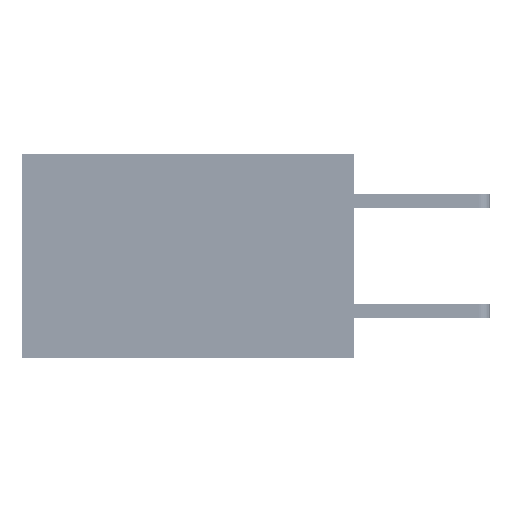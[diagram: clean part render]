
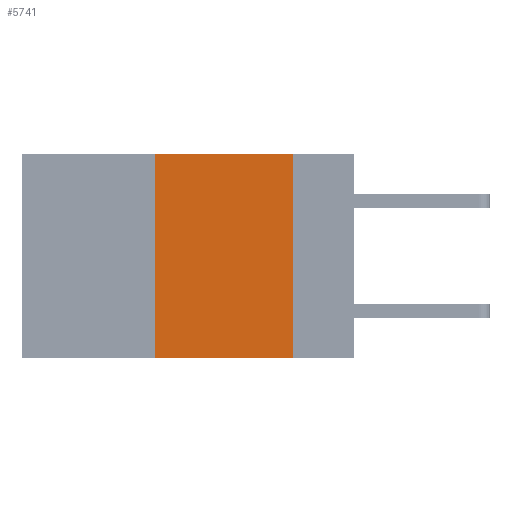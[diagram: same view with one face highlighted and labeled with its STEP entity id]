
A CAD part, left-side view. The second image highlights one B-rep face of the part: STEP entity #5741.
In plain terms, the highlighted planar face has unit normal (-1, 0, 0).
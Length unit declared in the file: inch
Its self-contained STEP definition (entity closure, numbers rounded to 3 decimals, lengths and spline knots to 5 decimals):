
#318 = EDGE_CURVE ( 'NONE', #2226, #13308, #30895, .T. ) ;
#563 = FACE_OUTER_BOUND ( 'NONE', #6860, .T. ) ;
#1146 = CARTESIAN_POINT ( 'NONE',  ( 0., 0.11, 0. ) ) ;
#2070 = AXIS2_PLACEMENT_3D ( 'NONE', #8874, #25288, #28802 ) ;
#2226 = VERTEX_POINT ( 'NONE', #36216 ) ;
#4583 = LINE ( 'NONE', #12927, #40667 ) ;
#5711 = ORIENTED_EDGE ( 'NONE', *, *, #24174, .T. ) ;
#5741 = ADVANCED_FACE ( 'NONE', ( #563 ), #32286, .F. ) ;
#6860 = EDGE_LOOP ( 'NONE', ( #35688, #47571, #44228, #5711 ) ) ;
#8874 = CARTESIAN_POINT ( 'NONE',  ( 0., 0.6, 0. ) ) ;
#10794 = CARTESIAN_POINT ( 'NONE',  ( 0., 0.11, -0.37 ) ) ;
#12927 = CARTESIAN_POINT ( 'NONE',  ( 0., 0.6, -0.37 ) ) ;
#13308 = VERTEX_POINT ( 'NONE', #1146 ) ;
#15041 = DIRECTION ( 'NONE',  ( 0., 0., 1. ) ) ;
#18506 = CARTESIAN_POINT ( 'NONE',  ( 0., 0.36, -0.37 ) ) ;
#19337 = CARTESIAN_POINT ( 'NONE',  ( 0., 0.6, 0. ) ) ;
#20428 = VECTOR ( 'NONE', #29364, 39.37008 ) ;
#24174 = EDGE_CURVE ( 'NONE', #38677, #51711, #4583, .T. ) ;
#24541 = EDGE_CURVE ( 'NONE', #38677, #2226, #27924, .T. ) ;
#25288 = DIRECTION ( 'NONE',  ( 1., 0., 0. ) ) ;
#27020 = EDGE_CURVE ( 'NONE', #13308, #51711, #49791, .T. ) ;
#27924 = LINE ( 'NONE', #35458, #31139 ) ;
#28802 = DIRECTION ( 'NONE',  ( 0., 0., -1. ) ) ;
#29364 = DIRECTION ( 'NONE',  ( 0., 0., -1. ) ) ;
#29579 = DIRECTION ( 'NONE',  ( 0., -1., 0. ) ) ;
#30895 = LINE ( 'NONE', #19337, #51021 ) ;
#31139 = VECTOR ( 'NONE', #15041, 39.37008 ) ;
#32286 = PLANE ( 'NONE',  #2070 ) ;
#35458 = CARTESIAN_POINT ( 'NONE',  ( 0., 0.36, 0. ) ) ;
#35688 = ORIENTED_EDGE ( 'NONE', *, *, #27020, .F. ) ;
#36216 = CARTESIAN_POINT ( 'NONE',  ( 0., 0.36, 0. ) ) ;
#38677 = VERTEX_POINT ( 'NONE', #18506 ) ;
#40667 = VECTOR ( 'NONE', #29579, 39.37008 ) ;
#41990 = CARTESIAN_POINT ( 'NONE',  ( 0., 0.11, 0. ) ) ;
#44228 = ORIENTED_EDGE ( 'NONE', *, *, #24541, .F. ) ;
#47571 = ORIENTED_EDGE ( 'NONE', *, *, #318, .F. ) ;
#49791 = LINE ( 'NONE', #41990, #20428 ) ;
#51021 = VECTOR ( 'NONE', #51067, 39.37008 ) ;
#51067 = DIRECTION ( 'NONE',  ( 0., -1., 0. ) ) ;
#51711 = VERTEX_POINT ( 'NONE', #10794 ) ;
